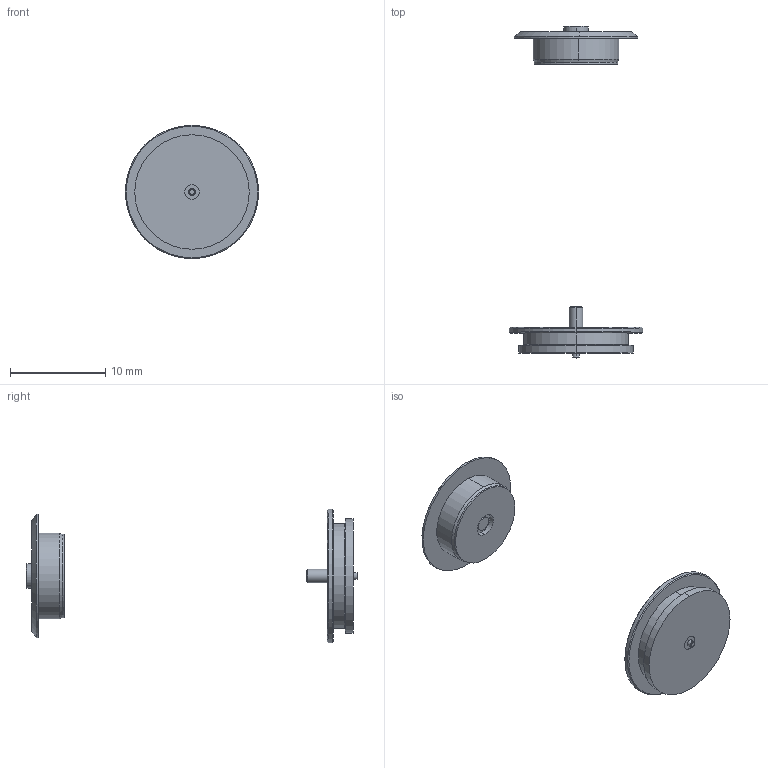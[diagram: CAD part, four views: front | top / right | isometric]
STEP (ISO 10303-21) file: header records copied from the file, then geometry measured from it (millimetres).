
FILE_DESCRIPTION (( 'STEP AP214' ), '1' );
FILE_NAME ('689N02229011F0E.STEP', '2023-07-26T20:52:22', ( '' ), ( '' ), 'SwSTEP 2.0', 'SolidWorks 2023', '' );
FILE_SCHEMA (( 'AUTOMOTIVE_DESIGN' ));
Length unit declared in the file: millimetre
Products named in the file (3): 686N02222011F0E; 689N02229011F0E; 685N0222P011F0E
Assembly tree (2 placements, depth 2):
  689N02229011F0E
    686N02222011F0E
    685N0222P011F0E
Bounding box: 14 x 34.82 x 14 mm (x, y, z)
Volume: 449.8 mm3; surface area: 880.9 mm2
Topology: 2 solids, 2 shells, 66 faces, 132 edges, 78 vertices
Faces by surface type: cylinder 30, cone 22, plane 14
Entity records: 1780 total; most frequent: DIRECTION 346, CARTESIAN_POINT 277, ORIENTED_EDGE 256, AXIS2_PLACEMENT_3D 147, EDGE_CURVE 128, VERTEX_POINT 78, EDGE_LOOP 78, CIRCLE 76
